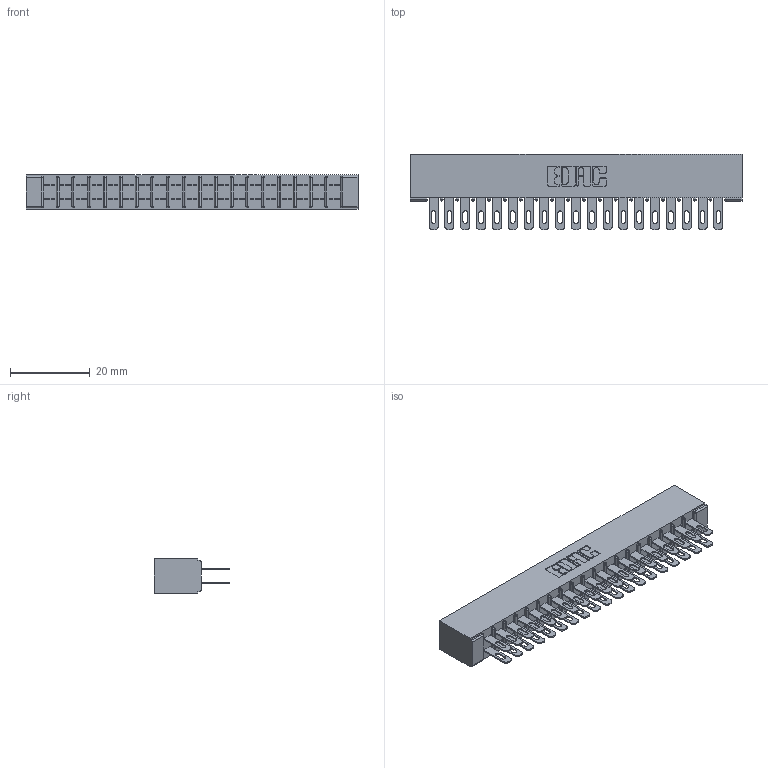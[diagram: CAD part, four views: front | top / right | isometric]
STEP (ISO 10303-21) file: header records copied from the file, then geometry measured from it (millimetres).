
FILE_DESCRIPTION (( 'STEP AP203' ), '1' );
FILE_NAME ('305-038-500-501.STEP', '2019-09-09T18:21:12', ( '' ), ( '' ), 'SwSTEP 2.0', 'SolidWorks 2016', '' );
FILE_SCHEMA (( 'CONFIG_CONTROL_DESIGN' ));
Length unit declared in the file: inch
Products named in the file (3): 305-290-001_500; 305 Part_No Mounting; 305-038-500-501
Assembly tree (39 placements, depth 2):
  305-038-500-501
    305 Part_No Mounting
    305-290-001_500  x38
Bounding box: 83.16 x 18.85 x 8.71 mm (x, y, z)
Volume: 5260.9 mm3; surface area: 11590.3 mm2
Topology: 39 solids, 39 shells, 2008 faces, 5745 edges, 3726 vertices
Faces by surface type: plane 1128, cylinder 804, sphere 76
Entity records: 23116 total; most frequent: CARTESIAN_POINT 3823, ORIENTED_EDGE 3790, DIRECTION 3717, EDGE_CURVE 1895, LINE 1509, VECTOR 1509, VERTEX_POINT 1210, AXIS2_PLACEMENT_3D 1104
